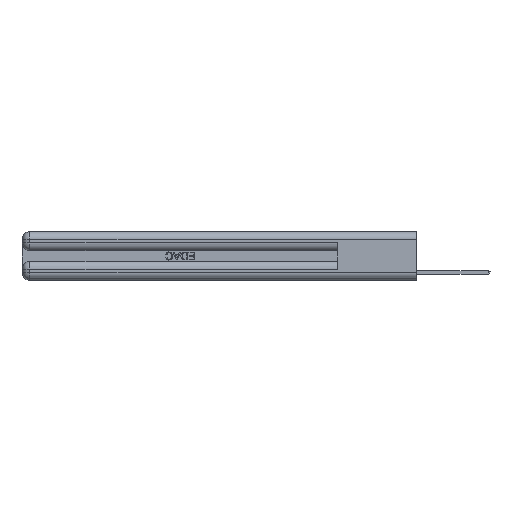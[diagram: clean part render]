
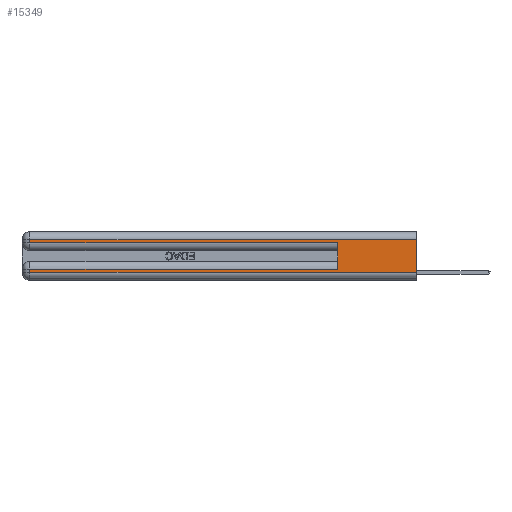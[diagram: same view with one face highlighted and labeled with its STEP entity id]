
A CAD part, left-side view. The second image highlights one B-rep face of the part: STEP entity #15349.
In plain terms, the highlighted planar face has unit normal (-1, 0, 0).
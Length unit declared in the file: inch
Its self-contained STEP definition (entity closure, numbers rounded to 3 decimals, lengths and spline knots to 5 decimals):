
#556 = ORIENTED_EDGE ( 'NONE', *, *, #15194, .F. ) ;
#1352 = ORIENTED_EDGE ( 'NONE', *, *, #4727, .T. ) ;
#2315 = DIRECTION ( 'NONE',  ( 0., -1., 0. ) ) ;
#2355 = VECTOR ( 'NONE', #7809, 39.37008 ) ;
#2788 = CARTESIAN_POINT ( 'NONE',  ( 0., 0., 0.31 ) ) ;
#3154 = VERTEX_POINT ( 'NONE', #30880 ) ;
#3439 = VERTEX_POINT ( 'NONE', #12642 ) ;
#3725 = VERTEX_POINT ( 'NONE', #15407 ) ;
#4727 = EDGE_CURVE ( 'NONE', #17121, #11859, #21476, .T. ) ;
#5017 = EDGE_CURVE ( 'NONE', #3154, #17121, #26333, .T. ) ;
#6398 = CARTESIAN_POINT ( 'NONE',  ( 0., 0., 0.285 ) ) ;
#6550 = ORIENTED_EDGE ( 'NONE', *, *, #29538, .F. ) ;
#6847 = PLANE ( 'NONE',  #25302 ) ;
#7809 = DIRECTION ( 'NONE',  ( 0., 0., -1. ) ) ;
#8398 = VECTOR ( 'NONE', #21027, 39.37008 ) ;
#8779 = CARTESIAN_POINT ( 'NONE',  ( 0., 0., 0.37 ) ) ;
#9718 = CARTESIAN_POINT ( 'NONE',  ( 0., 0.6, 0.145 ) ) ;
#10004 = CARTESIAN_POINT ( 'NONE',  ( 0., 2.94, 0.37 ) ) ;
#11640 = CARTESIAN_POINT ( 'NONE',  ( 0., 2.94, 0.06 ) ) ;
#11659 = VECTOR ( 'NONE', #32489, 39.37008 ) ;
#11754 = LINE ( 'NONE', #21081, #17897 ) ;
#11859 = VERTEX_POINT ( 'NONE', #21011 ) ;
#12497 = LINE ( 'NONE', #9718, #12885 ) ;
#12642 = CARTESIAN_POINT ( 'NONE',  ( 0., 0., 0.06 ) ) ;
#12670 = VERTEX_POINT ( 'NONE', #19469 ) ;
#12885 = VECTOR ( 'NONE', #22901, 39.37008 ) ;
#13277 = LINE ( 'NONE', #25911, #19398 ) ;
#13407 = EDGE_LOOP ( 'NONE', ( #556, #28939, #1352, #24815, #6550, #15879, #24114, #14832 ) ) ;
#13530 = VERTEX_POINT ( 'NONE', #32334 ) ;
#14832 = ORIENTED_EDGE ( 'NONE', *, *, #29731, .T. ) ;
#15194 = EDGE_CURVE ( 'NONE', #3154, #3439, #17500, .T. ) ;
#15349 = ADVANCED_FACE ( 'NONE', ( #33668 ), #6847, .F. ) ;
#15407 = CARTESIAN_POINT ( 'NONE',  ( 0., 0.6, 0.285 ) ) ;
#15879 = ORIENTED_EDGE ( 'NONE', *, *, #23096, .T. ) ;
#15904 = EDGE_CURVE ( 'NONE', #12670, #17842, #28873, .T. ) ;
#16951 = CARTESIAN_POINT ( 'NONE',  ( 0., 2.94, 0.37 ) ) ;
#17121 = VERTEX_POINT ( 'NONE', #31388 ) ;
#17500 = LINE ( 'NONE', #18419, #2355 ) ;
#17842 = VERTEX_POINT ( 'NONE', #11640 ) ;
#17897 = VECTOR ( 'NONE', #29049, 39.37008 ) ;
#18419 = CARTESIAN_POINT ( 'NONE',  ( 0., 0., 0.37 ) ) ;
#18611 = LINE ( 'NONE', #6398, #11659 ) ;
#19398 = VECTOR ( 'NONE', #2315, 39.37008 ) ;
#19469 = CARTESIAN_POINT ( 'NONE',  ( 0., 2.94, 0.085 ) ) ;
#21011 = CARTESIAN_POINT ( 'NONE',  ( 0., 2.94, 0.285 ) ) ;
#21027 = DIRECTION ( 'NONE',  ( 0., 1., 0. ) ) ;
#21081 = CARTESIAN_POINT ( 'NONE',  ( 0., 0., 0.085 ) ) ;
#21476 = LINE ( 'NONE', #16951, #30002 ) ;
#22441 = DIRECTION ( 'NONE',  ( 1., 0., 0. ) ) ;
#22901 = DIRECTION ( 'NONE',  ( 0., 0., 1. ) ) ;
#23096 = EDGE_CURVE ( 'NONE', #13530, #12670, #11754, .T. ) ;
#24114 = ORIENTED_EDGE ( 'NONE', *, *, #15904, .T. ) ;
#24815 = ORIENTED_EDGE ( 'NONE', *, *, #28648, .T. ) ;
#25302 = AXIS2_PLACEMENT_3D ( 'NONE', #8779, #22441, #26986 ) ;
#25911 = CARTESIAN_POINT ( 'NONE',  ( 0., 0., 0.06 ) ) ;
#26333 = LINE ( 'NONE', #2788, #8398 ) ;
#26986 = DIRECTION ( 'NONE',  ( 0., 0., -1. ) ) ;
#28648 = EDGE_CURVE ( 'NONE', #11859, #3725, #18611, .T. ) ;
#28656 = DIRECTION ( 'NONE',  ( 0., 0., -1. ) ) ;
#28873 = LINE ( 'NONE', #10004, #29253 ) ;
#28939 = ORIENTED_EDGE ( 'NONE', *, *, #5017, .T. ) ;
#29049 = DIRECTION ( 'NONE',  ( 0., 1., 0. ) ) ;
#29253 = VECTOR ( 'NONE', #28656, 39.37008 ) ;
#29538 = EDGE_CURVE ( 'NONE', #13530, #3725, #12497, .T. ) ;
#29731 = EDGE_CURVE ( 'NONE', #17842, #3439, #13277, .T. ) ;
#29992 = DIRECTION ( 'NONE',  ( 0., 0., -1. ) ) ;
#30002 = VECTOR ( 'NONE', #29992, 39.37008 ) ;
#30880 = CARTESIAN_POINT ( 'NONE',  ( 0., 0., 0.31 ) ) ;
#31388 = CARTESIAN_POINT ( 'NONE',  ( 0., 2.94, 0.31 ) ) ;
#32334 = CARTESIAN_POINT ( 'NONE',  ( 0., 0.6, 0.085 ) ) ;
#32489 = DIRECTION ( 'NONE',  ( 0., -1., 0. ) ) ;
#33668 = FACE_OUTER_BOUND ( 'NONE', #13407, .T. ) ;
